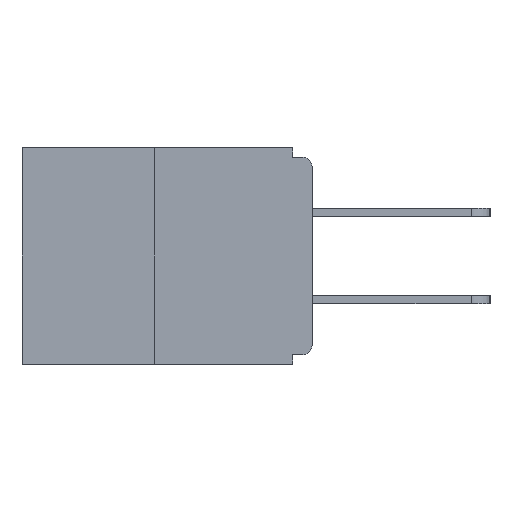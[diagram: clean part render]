
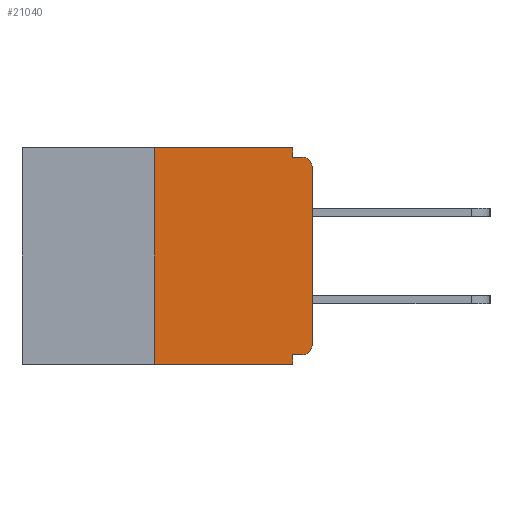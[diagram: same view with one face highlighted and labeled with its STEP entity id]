
A CAD part, left-side view. The second image highlights one B-rep face of the part: STEP entity #21040.
In plain terms, the highlighted planar face has unit normal (-1, 0, 0).
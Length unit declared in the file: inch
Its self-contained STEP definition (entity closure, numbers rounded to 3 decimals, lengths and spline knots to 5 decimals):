
#172 = CARTESIAN_POINT ( 'NONE',  ( 0., 0.031, 0. ) ) ;
#493 = VECTOR ( 'NONE', #17670, 39.37008 ) ;
#943 = EDGE_CURVE ( 'NONE', #7597, #14366, #16207, .T. ) ;
#972 = CARTESIAN_POINT ( 'NONE',  ( 0., 0., 0. ) ) ;
#1117 = ORIENTED_EDGE ( 'NONE', *, *, #19889, .F. ) ;
#1283 = LINE ( 'NONE', #15409, #12134 ) ;
#1285 = CARTESIAN_POINT ( 'NONE',  ( 0., 0.46, 0. ) ) ;
#1695 = DIRECTION ( 'NONE',  ( 0., 0., -1. ) ) ;
#2095 = CARTESIAN_POINT ( 'NONE',  ( 0., 0.031, 0. ) ) ;
#2492 = DIRECTION ( 'NONE',  ( 0., 0., -1. ) ) ;
#2723 = VERTEX_POINT ( 'NONE', #9235 ) ;
#2789 = VERTEX_POINT ( 'NONE', #4156 ) ;
#2863 = CARTESIAN_POINT ( 'NONE',  ( 0., 0.46, -0.343 ) ) ;
#3539 = LINE ( 'NONE', #20696, #21448 ) ;
#3782 = LINE ( 'NONE', #9452, #10784 ) ;
#3958 = DIRECTION ( 'NONE',  ( 0., 0., 1. ) ) ;
#4042 = ORIENTED_EDGE ( 'NONE', *, *, #18170, .F. ) ;
#4156 = CARTESIAN_POINT ( 'NONE',  ( 0., 0.25, -0.343 ) ) ;
#4832 = DIRECTION ( 'NONE',  ( 0., 1., 0. ) ) ;
#4987 = PLANE ( 'NONE',  #23016 ) ;
#5522 = LINE ( 'NONE', #972, #493 ) ;
#5642 = VECTOR ( 'NONE', #13849, 39.37008 ) ;
#6609 = VERTEX_POINT ( 'NONE', #14503 ) ;
#6708 = EDGE_CURVE ( 'NONE', #14923, #18447, #13318, .T. ) ;
#7597 = VERTEX_POINT ( 'NONE', #19824 ) ;
#7845 = CARTESIAN_POINT ( 'NONE',  ( 0., 0.015, -0.313 ) ) ;
#8061 = VECTOR ( 'NONE', #19777, 39.37008 ) ;
#8971 = EDGE_CURVE ( 'NONE', #2789, #2723, #3782, .T. ) ;
#9022 = VERTEX_POINT ( 'NONE', #9599 ) ;
#9235 = CARTESIAN_POINT ( 'NONE',  ( 0., 0.25, 0. ) ) ;
#9250 = EDGE_CURVE ( 'NONE', #23609, #6609, #5522, .T. ) ;
#9382 = VERTEX_POINT ( 'NONE', #22613 ) ;
#9452 = CARTESIAN_POINT ( 'NONE',  ( 0., 0.25, 0. ) ) ;
#9476 = CARTESIAN_POINT ( 'NONE',  ( 0., 0.015, -0.03 ) ) ;
#9561 = CARTESIAN_POINT ( 'NONE',  ( 0., 0., -0.313 ) ) ;
#9599 = CARTESIAN_POINT ( 'NONE',  ( 0., 0.015, -0.015 ) ) ;
#9805 = LINE ( 'NONE', #2863, #8061 ) ;
#9989 = DIRECTION ( 'NONE',  ( 0., 0., -1. ) ) ;
#10092 = AXIS2_PLACEMENT_3D ( 'NONE', #7845, #21205, #2492 ) ;
#10530 = AXIS2_PLACEMENT_3D ( 'NONE', #9476, #12946, #1695 ) ;
#10629 = LINE ( 'NONE', #23197, #5642 ) ;
#10642 = CIRCLE ( 'NONE', #10530, 0.015 ) ;
#10737 = EDGE_CURVE ( 'NONE', #2789, #14366, #9805, .T. ) ;
#10784 = VECTOR ( 'NONE', #3958, 39.37008 ) ;
#11269 = DIRECTION ( 'NONE',  ( 0., 0., -1. ) ) ;
#11327 = DIRECTION ( 'NONE',  ( 0., 0., -1. ) ) ;
#11945 = CARTESIAN_POINT ( 'NONE',  ( 0., 0.031, -0.343 ) ) ;
#12134 = VECTOR ( 'NONE', #4832, 39.37008 ) ;
#12946 = DIRECTION ( 'NONE',  ( -1., 0., 0. ) ) ;
#13318 = LINE ( 'NONE', #172, #15040 ) ;
#13849 = DIRECTION ( 'NONE',  ( 0., -1., 0. ) ) ;
#14366 = VERTEX_POINT ( 'NONE', #11945 ) ;
#14503 = CARTESIAN_POINT ( 'NONE',  ( 0., 0., -0.03 ) ) ;
#14923 = VERTEX_POINT ( 'NONE', #2095 ) ;
#14926 = DIRECTION ( 'NONE',  ( 1., 0., 0. ) ) ;
#15040 = VECTOR ( 'NONE', #11327, 39.37008 ) ;
#15136 = DIRECTION ( 'NONE',  ( 0., -1., 0. ) ) ;
#15259 = ORIENTED_EDGE ( 'NONE', *, *, #8971, .F. ) ;
#15409 = CARTESIAN_POINT ( 'NONE',  ( 0., 0., -0.328 ) ) ;
#15854 = CARTESIAN_POINT ( 'NONE',  ( 0., 0.031, -0.343 ) ) ;
#15890 = EDGE_LOOP ( 'NONE', ( #20469, #15259, #22009, #21622, #1117, #19556, #18262, #21520, #4042, #20852 ) ) ;
#16207 = LINE ( 'NONE', #15854, #19408 ) ;
#16693 = EDGE_CURVE ( 'NONE', #6609, #9022, #10642, .T. ) ;
#17670 = DIRECTION ( 'NONE',  ( 0., 0., 1. ) ) ;
#18170 = EDGE_CURVE ( 'NONE', #18447, #9022, #3539, .T. ) ;
#18262 = ORIENTED_EDGE ( 'NONE', *, *, #9250, .T. ) ;
#18447 = VERTEX_POINT ( 'NONE', #19999 ) ;
#19408 = VECTOR ( 'NONE', #9989, 39.37008 ) ;
#19556 = ORIENTED_EDGE ( 'NONE', *, *, #20126, .T. ) ;
#19777 = DIRECTION ( 'NONE',  ( 0., -1., 0. ) ) ;
#19824 = CARTESIAN_POINT ( 'NONE',  ( 0., 0.031, -0.328 ) ) ;
#19889 = EDGE_CURVE ( 'NONE', #9382, #7597, #1283, .T. ) ;
#19999 = CARTESIAN_POINT ( 'NONE',  ( 0., 0.031, -0.015 ) ) ;
#20126 = EDGE_CURVE ( 'NONE', #9382, #23609, #21261, .T. ) ;
#20469 = ORIENTED_EDGE ( 'NONE', *, *, #21363, .F. ) ;
#20696 = CARTESIAN_POINT ( 'NONE',  ( 0., 0., -0.015 ) ) ;
#20852 = ORIENTED_EDGE ( 'NONE', *, *, #6708, .F. ) ;
#20918 = FACE_OUTER_BOUND ( 'NONE', #15890, .T. ) ;
#21040 = ADVANCED_FACE ( 'NONE', ( #20918 ), #4987, .F. ) ;
#21205 = DIRECTION ( 'NONE',  ( -1., 0., 0. ) ) ;
#21261 = CIRCLE ( 'NONE', #10092, 0.015 ) ;
#21363 = EDGE_CURVE ( 'NONE', #2723, #14923, #10629, .T. ) ;
#21448 = VECTOR ( 'NONE', #15136, 39.37008 ) ;
#21520 = ORIENTED_EDGE ( 'NONE', *, *, #16693, .T. ) ;
#21622 = ORIENTED_EDGE ( 'NONE', *, *, #943, .F. ) ;
#22009 = ORIENTED_EDGE ( 'NONE', *, *, #10737, .T. ) ;
#22613 = CARTESIAN_POINT ( 'NONE',  ( 0., 0.015, -0.328 ) ) ;
#23016 = AXIS2_PLACEMENT_3D ( 'NONE', #1285, #14926, #11269 ) ;
#23197 = CARTESIAN_POINT ( 'NONE',  ( 0., 0.46, 0. ) ) ;
#23609 = VERTEX_POINT ( 'NONE', #9561 ) ;
